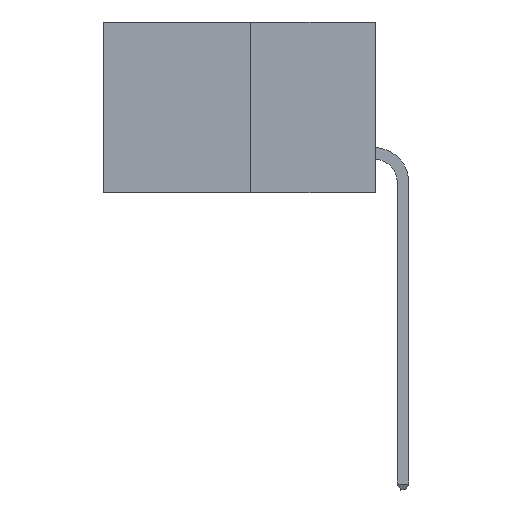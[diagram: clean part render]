
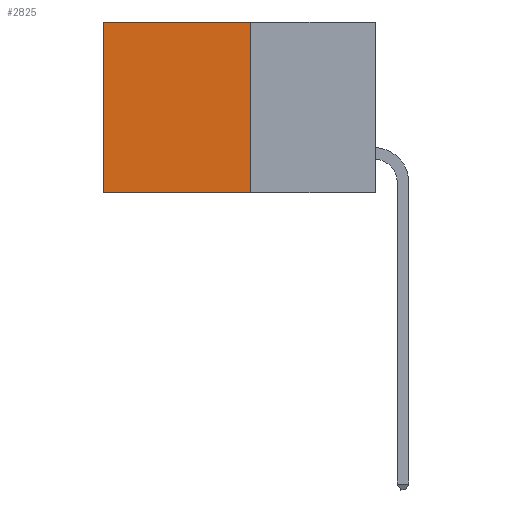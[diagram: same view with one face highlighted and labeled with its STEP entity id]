
A CAD part, left-side view. The second image highlights one B-rep face of the part: STEP entity #2825.
In plain terms, the highlighted planar face has unit normal (-1, 0, 0).
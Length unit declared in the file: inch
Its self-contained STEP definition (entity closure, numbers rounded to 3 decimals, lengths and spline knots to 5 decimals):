
#50 = EDGE_CURVE ( 'NONE', #9225, #1605, #7974, .T. ) ;
#468 = EDGE_CURVE ( 'NONE', #1605, #4234, #12731, .T. ) ;
#625 = AXIS2_PLACEMENT_3D ( 'NONE', #6939, #4539, #7287 ) ;
#784 = EDGE_CURVE ( 'NONE', #9225, #10776, #9930, .T. ) ;
#1603 = CARTESIAN_POINT ( 'NONE',  ( 0.277, 0.27, -0.37 ) ) ;
#1605 = VERTEX_POINT ( 'NONE', #13802 ) ;
#1864 = DIRECTION ( 'NONE',  ( 0., 1., 0. ) ) ;
#2825 = ADVANCED_FACE ( 'NONE', ( #11207 ), #7072, .F. ) ;
#2865 = CARTESIAN_POINT ( 'NONE',  ( 0.277, 0.59, -0.37 ) ) ;
#3267 = EDGE_CURVE ( 'NONE', #10776, #4234, #10342, .T. ) ;
#3456 = CARTESIAN_POINT ( 'NONE',  ( 0.277, 0.27, 0. ) ) ;
#4234 = VERTEX_POINT ( 'NONE', #12376 ) ;
#4539 = DIRECTION ( 'NONE',  ( 1., 0., 0. ) ) ;
#5034 = DIRECTION ( 'NONE',  ( 0., 0., -1. ) ) ;
#5321 = CARTESIAN_POINT ( 'NONE',  ( 0.277, 0.59, 0. ) ) ;
#6724 = CARTESIAN_POINT ( 'NONE',  ( 0.277, 0.27, 0. ) ) ;
#6742 = VECTOR ( 'NONE', #9938, 39.37008 ) ;
#6939 = CARTESIAN_POINT ( 'NONE',  ( 0.277, 0.27, -0.37 ) ) ;
#7072 = PLANE ( 'NONE',  #625 ) ;
#7119 = EDGE_LOOP ( 'NONE', ( #8603, #8673, #9439, #9564 ) ) ;
#7287 = DIRECTION ( 'NONE',  ( 0., 0., -1. ) ) ;
#7662 = VECTOR ( 'NONE', #5034, 39.37008 ) ;
#7974 = LINE ( 'NONE', #9435, #7662 ) ;
#8246 = DIRECTION ( 'NONE',  ( 0., 0., -1. ) ) ;
#8603 = ORIENTED_EDGE ( 'NONE', *, *, #3267, .T. ) ;
#8673 = ORIENTED_EDGE ( 'NONE', *, *, #468, .F. ) ;
#9225 = VERTEX_POINT ( 'NONE', #6724 ) ;
#9435 = CARTESIAN_POINT ( 'NONE',  ( 0.277, 0.27, -0.37 ) ) ;
#9439 = ORIENTED_EDGE ( 'NONE', *, *, #50, .F. ) ;
#9564 = ORIENTED_EDGE ( 'NONE', *, *, #784, .T. ) ;
#9777 = VECTOR ( 'NONE', #1864, 39.37008 ) ;
#9930 = LINE ( 'NONE', #3456, #6742 ) ;
#9938 = DIRECTION ( 'NONE',  ( 0., 1., 0. ) ) ;
#10011 = VECTOR ( 'NONE', #8246, 39.37008 ) ;
#10342 = LINE ( 'NONE', #2865, #10011 ) ;
#10776 = VERTEX_POINT ( 'NONE', #5321 ) ;
#11207 = FACE_OUTER_BOUND ( 'NONE', #7119, .T. ) ;
#12376 = CARTESIAN_POINT ( 'NONE',  ( 0.277, 0.59, -0.37 ) ) ;
#12731 = LINE ( 'NONE', #1603, #9777 ) ;
#13802 = CARTESIAN_POINT ( 'NONE',  ( 0.277, 0.27, -0.37 ) ) ;
